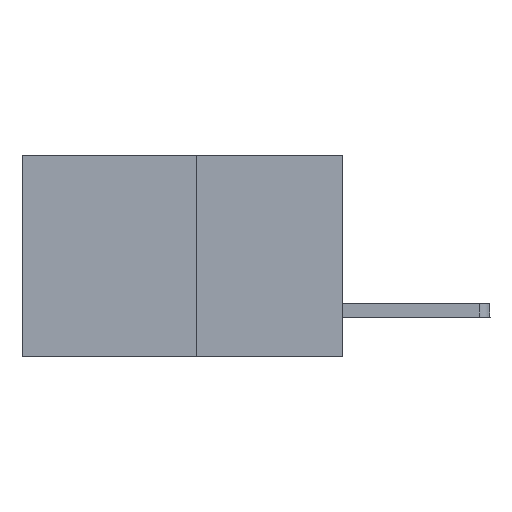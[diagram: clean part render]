
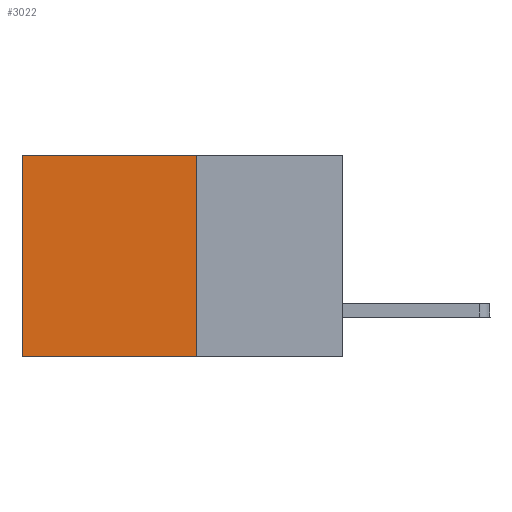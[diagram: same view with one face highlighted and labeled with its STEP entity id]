
A CAD part, left-side view. The second image highlights one B-rep face of the part: STEP entity #3022.
In plain terms, the highlighted planar face has unit normal (-1, 0, 0).
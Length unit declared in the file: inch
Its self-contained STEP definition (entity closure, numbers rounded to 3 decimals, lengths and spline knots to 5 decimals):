
#48 = VERTEX_POINT ( 'NONE', #4896 ) ;
#257 = CARTESIAN_POINT ( 'NONE',  ( 0.277, 0.27, 0. ) ) ;
#278 = CARTESIAN_POINT ( 'NONE',  ( 0.277, 0.27, 0. ) ) ;
#827 = ORIENTED_EDGE ( 'NONE', *, *, #8418, .T. ) ;
#915 = VECTOR ( 'NONE', #5381, 39.37008 ) ;
#1551 = VERTEX_POINT ( 'NONE', #2186 ) ;
#1669 = VECTOR ( 'NONE', #2255, 39.37008 ) ;
#1689 = VERTEX_POINT ( 'NONE', #278 ) ;
#1947 = EDGE_CURVE ( 'NONE', #1689, #48, #6302, .T. ) ;
#2186 = CARTESIAN_POINT ( 'NONE',  ( 0.277, 0.59, 0. ) ) ;
#2255 = DIRECTION ( 'NONE',  ( 0., 0., -1. ) ) ;
#2500 = EDGE_LOOP ( 'NONE', ( #827, #6389, #4967, #3712 ) ) ;
#2508 = LINE ( 'NONE', #4542, #2739 ) ;
#2739 = VECTOR ( 'NONE', #7947, 39.37008 ) ;
#2825 = LINE ( 'NONE', #257, #6060 ) ;
#2910 = CARTESIAN_POINT ( 'NONE',  ( 0.277, 0.27, -0.37 ) ) ;
#3018 = DIRECTION ( 'NONE',  ( 1., 0., 0. ) ) ;
#3022 = ADVANCED_FACE ( 'NONE', ( #3750 ), #7762, .F. ) ;
#3712 = ORIENTED_EDGE ( 'NONE', *, *, #6276, .T. ) ;
#3750 = FACE_OUTER_BOUND ( 'NONE', #2500, .T. ) ;
#4542 = CARTESIAN_POINT ( 'NONE',  ( 0.277, 0.59, -0.37 ) ) ;
#4896 = CARTESIAN_POINT ( 'NONE',  ( 0.277, 0.27, -0.37 ) ) ;
#4967 = ORIENTED_EDGE ( 'NONE', *, *, #1947, .F. ) ;
#4968 = DIRECTION ( 'NONE',  ( 0., 0., -1. ) ) ;
#5381 = DIRECTION ( 'NONE',  ( 0., 1., 0. ) ) ;
#5473 = LINE ( 'NONE', #6264, #915 ) ;
#5585 = CARTESIAN_POINT ( 'NONE',  ( 0.277, 0.59, -0.37 ) ) ;
#6060 = VECTOR ( 'NONE', #6787, 39.37008 ) ;
#6188 = EDGE_CURVE ( 'NONE', #48, #6602, #5473, .T. ) ;
#6264 = CARTESIAN_POINT ( 'NONE',  ( 0.277, 0.27, -0.37 ) ) ;
#6276 = EDGE_CURVE ( 'NONE', #1689, #1551, #2825, .T. ) ;
#6302 = LINE ( 'NONE', #2910, #1669 ) ;
#6389 = ORIENTED_EDGE ( 'NONE', *, *, #6188, .F. ) ;
#6405 = CARTESIAN_POINT ( 'NONE',  ( 0.277, 0.27, -0.37 ) ) ;
#6602 = VERTEX_POINT ( 'NONE', #5585 ) ;
#6787 = DIRECTION ( 'NONE',  ( 0., 1., 0. ) ) ;
#7728 = AXIS2_PLACEMENT_3D ( 'NONE', #6405, #3018, #4968 ) ;
#7762 = PLANE ( 'NONE',  #7728 ) ;
#7947 = DIRECTION ( 'NONE',  ( 0., 0., -1. ) ) ;
#8418 = EDGE_CURVE ( 'NONE', #1551, #6602, #2508, .T. ) ;
